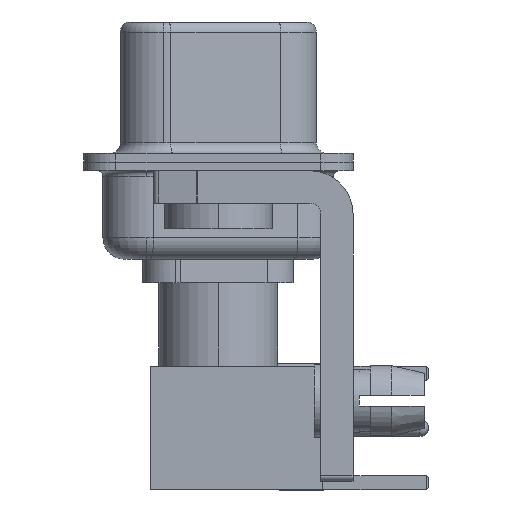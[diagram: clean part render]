
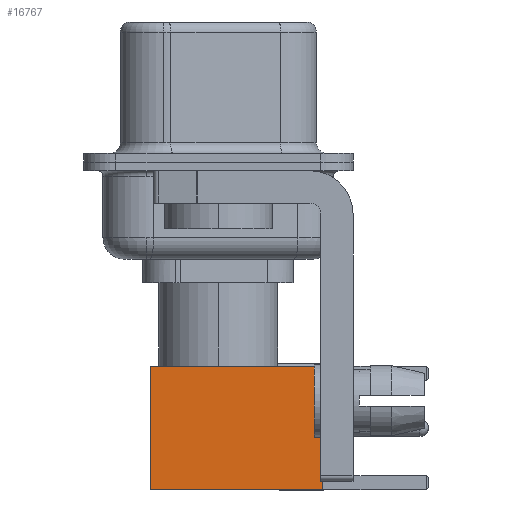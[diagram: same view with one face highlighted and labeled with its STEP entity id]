
A CAD part, left-side view. The second image highlights one B-rep face of the part: STEP entity #16767.
In plain terms, the highlighted face is planar.
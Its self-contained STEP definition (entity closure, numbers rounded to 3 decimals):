
#825 = ORIENTED_EDGE ( 'NONE', *, *, #25599, .F. ) ;
#3129 = EDGE_CURVE ( 'NONE', #25378, #28563, #25321, .T. ) ;
#3228 = CARTESIAN_POINT ( 'NONE',  ( -2.875, 2.875, 0. ) ) ;
#3761 = LINE ( 'NONE', #3228, #28297 ) ;
#4591 = EDGE_CURVE ( 'NONE', #25378, #29308, #5219, .T. ) ;
#5219 = LINE ( 'NONE', #27069, #33742 ) ;
#5568 = CARTESIAN_POINT ( 'NONE',  ( 2.875, 2.875, 8. ) ) ;
#9204 = VECTOR ( 'NONE', #27991, 1000. ) ;
#9217 = CARTESIAN_POINT ( 'NONE',  ( -2.875, 2.875, 0. ) ) ;
#9220 = VECTOR ( 'NONE', #34420, 1000. ) ;
#9267 = ORIENTED_EDGE ( 'NONE', *, *, #3129, .F. ) ;
#9428 = DIRECTION ( 'NONE',  ( 0., 0., 1. ) ) ;
#10340 = ORIENTED_EDGE ( 'NONE', *, *, #21525, .T. ) ;
#11304 = DIRECTION ( 'NONE',  ( 0., 0., -1. ) ) ;
#11395 = AXIS2_PLACEMENT_3D ( 'NONE', #17475, #25696, #9428 ) ;
#16161 = CARTESIAN_POINT ( 'NONE',  ( -2.875, 2.875, 8. ) ) ;
#16767 = ADVANCED_FACE ( 'NONE', ( #31088 ), #33965, .T. ) ;
#17475 = CARTESIAN_POINT ( 'NONE',  ( 2.875, 2.875, 0. ) ) ;
#17945 = CARTESIAN_POINT ( 'NONE',  ( 0., 2.875, 0. ) ) ;
#21525 = EDGE_CURVE ( 'NONE', #29308, #35377, #25099, .T. ) ;
#25099 = LINE ( 'NONE', #17945, #9220 ) ;
#25321 = LINE ( 'NONE', #33559, #9204 ) ;
#25378 = VERTEX_POINT ( 'NONE', #5568 ) ;
#25599 = EDGE_CURVE ( 'NONE', #28563, #35377, #3761, .T. ) ;
#25696 = DIRECTION ( 'NONE',  ( 0., 1., 0. ) ) ;
#27069 = CARTESIAN_POINT ( 'NONE',  ( 2.875, 2.875, 0. ) ) ;
#27991 = DIRECTION ( 'NONE',  ( -1., 0., 0. ) ) ;
#28297 = VECTOR ( 'NONE', #11304, 1000. ) ;
#28563 = VERTEX_POINT ( 'NONE', #16161 ) ;
#29308 = VERTEX_POINT ( 'NONE', #31684 ) ;
#29751 = DIRECTION ( 'NONE',  ( 0., 0., -1. ) ) ;
#30803 = EDGE_LOOP ( 'NONE', ( #32201, #10340, #825, #9267 ) ) ;
#31088 = FACE_OUTER_BOUND ( 'NONE', #30803, .T. ) ;
#31684 = CARTESIAN_POINT ( 'NONE',  ( 2.875, 2.875, 0. ) ) ;
#32201 = ORIENTED_EDGE ( 'NONE', *, *, #4591, .T. ) ;
#33559 = CARTESIAN_POINT ( 'NONE',  ( 0., 2.875, 8. ) ) ;
#33742 = VECTOR ( 'NONE', #29751, 1000. ) ;
#33965 = PLANE ( 'NONE',  #11395 ) ;
#34420 = DIRECTION ( 'NONE',  ( -1., 0., 0. ) ) ;
#35377 = VERTEX_POINT ( 'NONE', #9217 ) ;
